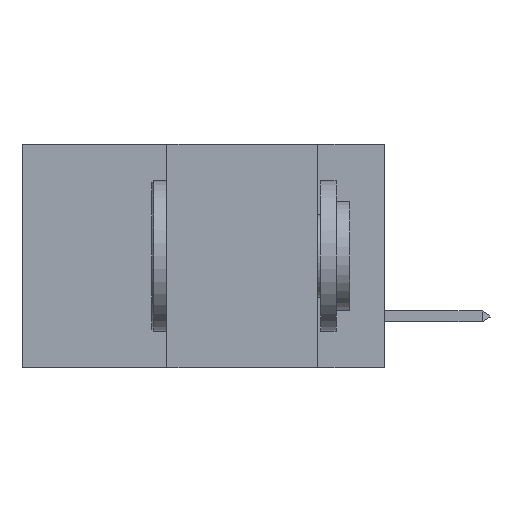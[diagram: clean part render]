
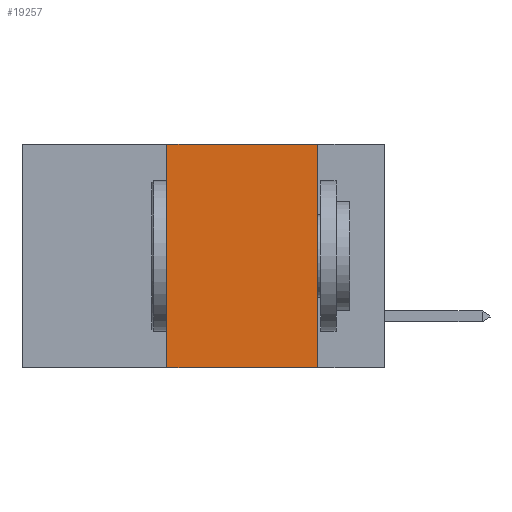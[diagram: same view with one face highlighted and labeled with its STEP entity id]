
A CAD part, left-side view. The second image highlights one B-rep face of the part: STEP entity #19257.
In plain terms, the highlighted planar face has unit normal (-1, 0, 0).
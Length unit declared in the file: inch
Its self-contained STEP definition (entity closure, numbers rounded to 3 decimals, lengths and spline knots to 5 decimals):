
#418 = CARTESIAN_POINT ( 'NONE',  ( 0., 0.36, 0. ) ) ;
#1707 = LINE ( 'NONE', #22537, #27108 ) ;
#3680 = DIRECTION ( 'NONE',  ( 0., -1., 0. ) ) ;
#3867 = DIRECTION ( 'NONE',  ( 0., 0., -1. ) ) ;
#3986 = EDGE_LOOP ( 'NONE', ( #21723, #13575, #7370, #4174 ) ) ;
#4174 = ORIENTED_EDGE ( 'NONE', *, *, #31174, .T. ) ;
#4830 = PLANE ( 'NONE',  #22439 ) ;
#5628 = LINE ( 'NONE', #16229, #31063 ) ;
#7370 = ORIENTED_EDGE ( 'NONE', *, *, #10652, .F. ) ;
#8345 = VERTEX_POINT ( 'NONE', #26113 ) ;
#9716 = VERTEX_POINT ( 'NONE', #31668 ) ;
#10652 = EDGE_CURVE ( 'NONE', #8345, #16648, #1707, .T. ) ;
#11972 = EDGE_CURVE ( 'NONE', #16648, #20889, #5628, .T. ) ;
#12272 = EDGE_CURVE ( 'NONE', #20889, #9716, #20297, .T. ) ;
#12973 = VECTOR ( 'NONE', #3867, 39.37008 ) ;
#13575 = ORIENTED_EDGE ( 'NONE', *, *, #11972, .F. ) ;
#13656 = CARTESIAN_POINT ( 'NONE',  ( 0., 0.11, 0. ) ) ;
#14597 = FACE_OUTER_BOUND ( 'NONE', #3986, .T. ) ;
#16229 = CARTESIAN_POINT ( 'NONE',  ( 0., 0.6, 0. ) ) ;
#16648 = VERTEX_POINT ( 'NONE', #418 ) ;
#17166 = DIRECTION ( 'NONE',  ( 1., 0., 0. ) ) ;
#17351 = VECTOR ( 'NONE', #24243, 39.37008 ) ;
#19257 = ADVANCED_FACE ( 'NONE', ( #14597 ), #4830, .F. ) ;
#19617 = CARTESIAN_POINT ( 'NONE',  ( 0., 0.6, 0. ) ) ;
#19650 = LINE ( 'NONE', #26603, #17351 ) ;
#20297 = LINE ( 'NONE', #30876, #12973 ) ;
#20889 = VERTEX_POINT ( 'NONE', #13656 ) ;
#21723 = ORIENTED_EDGE ( 'NONE', *, *, #12272, .F. ) ;
#22439 = AXIS2_PLACEMENT_3D ( 'NONE', #19617, #17166, #29591 ) ;
#22537 = CARTESIAN_POINT ( 'NONE',  ( 0., 0.36, 0. ) ) ;
#24243 = DIRECTION ( 'NONE',  ( 0., -1., 0. ) ) ;
#25262 = DIRECTION ( 'NONE',  ( 0., 0., 1. ) ) ;
#26113 = CARTESIAN_POINT ( 'NONE',  ( 0., 0.36, -0.37 ) ) ;
#26603 = CARTESIAN_POINT ( 'NONE',  ( 0., 0.6, -0.37 ) ) ;
#27108 = VECTOR ( 'NONE', #25262, 39.37008 ) ;
#29591 = DIRECTION ( 'NONE',  ( 0., 0., -1. ) ) ;
#30876 = CARTESIAN_POINT ( 'NONE',  ( 0., 0.11, 0. ) ) ;
#31063 = VECTOR ( 'NONE', #3680, 39.37008 ) ;
#31174 = EDGE_CURVE ( 'NONE', #8345, #9716, #19650, .T. ) ;
#31668 = CARTESIAN_POINT ( 'NONE',  ( 0., 0.11, -0.37 ) ) ;
